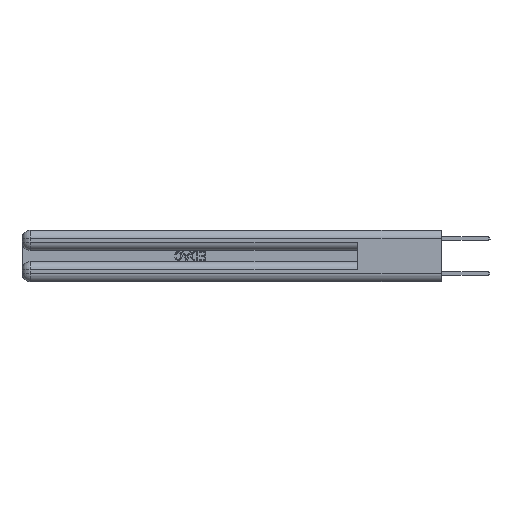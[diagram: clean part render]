
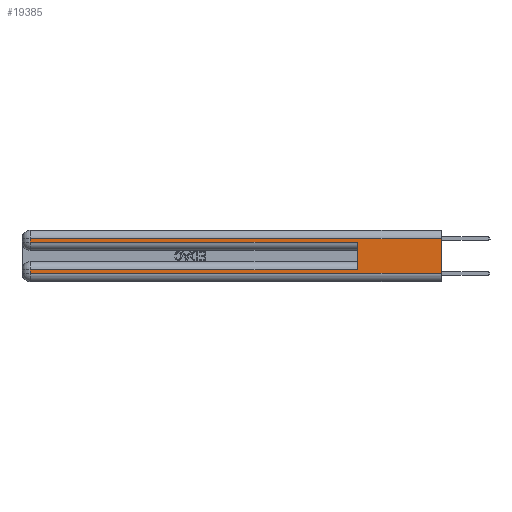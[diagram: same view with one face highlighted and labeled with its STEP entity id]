
A CAD part, left-side view. The second image highlights one B-rep face of the part: STEP entity #19385.
In plain terms, the highlighted planar face has unit normal (-1, 0, 0).
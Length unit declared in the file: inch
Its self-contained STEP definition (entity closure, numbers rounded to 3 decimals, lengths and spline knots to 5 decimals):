
#623 = CARTESIAN_POINT ( 'NONE',  ( 0., 0., 0.31 ) ) ;
#928 = ORIENTED_EDGE ( 'NONE', *, *, #11760, .T. ) ;
#1176 = LINE ( 'NONE', #1512, #12328 ) ;
#1384 = VERTEX_POINT ( 'NONE', #2148 ) ;
#1512 = CARTESIAN_POINT ( 'NONE',  ( 0., 2.94, 0.37 ) ) ;
#1855 = EDGE_CURVE ( 'NONE', #19437, #6624, #1176, .T. ) ;
#2148 = CARTESIAN_POINT ( 'NONE',  ( 0., 2.94, 0.085 ) ) ;
#2198 = DIRECTION ( 'NONE',  ( 0., 0., -1. ) ) ;
#2955 = DIRECTION ( 'NONE',  ( 0., 0., 1. ) ) ;
#3043 = ORIENTED_EDGE ( 'NONE', *, *, #7144, .T. ) ;
#3128 = FACE_OUTER_BOUND ( 'NONE', #19360, .T. ) ;
#3253 = ORIENTED_EDGE ( 'NONE', *, *, #17831, .F. ) ;
#3725 = DIRECTION ( 'NONE',  ( 0., 0., -1. ) ) ;
#3850 = VECTOR ( 'NONE', #22879, 39.37008 ) ;
#3863 = VERTEX_POINT ( 'NONE', #15389 ) ;
#3916 = LINE ( 'NONE', #19191, #9320 ) ;
#4671 = EDGE_CURVE ( 'NONE', #19615, #22689, #10793, .T. ) ;
#4676 = VECTOR ( 'NONE', #3725, 39.37008 ) ;
#4819 = ORIENTED_EDGE ( 'NONE', *, *, #1855, .T. ) ;
#6213 = CARTESIAN_POINT ( 'NONE',  ( 0., 0., 0.06 ) ) ;
#6471 = EDGE_CURVE ( 'NONE', #19615, #19437, #17158, .T. ) ;
#6624 = VERTEX_POINT ( 'NONE', #20461 ) ;
#7003 = CARTESIAN_POINT ( 'NONE',  ( 0., 2.94, 0.37 ) ) ;
#7045 = VECTOR ( 'NONE', #2198, 39.37008 ) ;
#7063 = EDGE_CURVE ( 'NONE', #12581, #22689, #22106, .T. ) ;
#7144 = EDGE_CURVE ( 'NONE', #1384, #12581, #22788, .T. ) ;
#8140 = VECTOR ( 'NONE', #27107, 39.37008 ) ;
#9320 = VECTOR ( 'NONE', #2955, 39.37008 ) ;
#9413 = VECTOR ( 'NONE', #19234, 39.37008 ) ;
#9540 = CARTESIAN_POINT ( 'NONE',  ( 0., 0., 0.085 ) ) ;
#10793 = LINE ( 'NONE', #12842, #4676 ) ;
#10964 = DIRECTION ( 'NONE',  ( 0., 0., -1. ) ) ;
#11760 = EDGE_CURVE ( 'NONE', #6624, #3863, #24926, .T. ) ;
#12117 = ORIENTED_EDGE ( 'NONE', *, *, #22693, .T. ) ;
#12328 = VECTOR ( 'NONE', #10964, 39.37008 ) ;
#12581 = VERTEX_POINT ( 'NONE', #21382 ) ;
#12842 = CARTESIAN_POINT ( 'NONE',  ( 0., 0., 0.37 ) ) ;
#13700 = ORIENTED_EDGE ( 'NONE', *, *, #7063, .T. ) ;
#15389 = CARTESIAN_POINT ( 'NONE',  ( 0., 0.6, 0.285 ) ) ;
#15562 = LINE ( 'NONE', #9540, #9413 ) ;
#15991 = DIRECTION ( 'NONE',  ( 1., 0., 0. ) ) ;
#16040 = CARTESIAN_POINT ( 'NONE',  ( 0., 0., 0.285 ) ) ;
#16197 = CARTESIAN_POINT ( 'NONE',  ( 0., 0., 0.37 ) ) ;
#17158 = LINE ( 'NONE', #29206, #8140 ) ;
#17831 = EDGE_CURVE ( 'NONE', #28899, #3863, #3916, .T. ) ;
#18501 = DIRECTION ( 'NONE',  ( 0., 0., -1. ) ) ;
#19032 = ORIENTED_EDGE ( 'NONE', *, *, #4671, .F. ) ;
#19191 = CARTESIAN_POINT ( 'NONE',  ( 0., 0.6, 0.145 ) ) ;
#19234 = DIRECTION ( 'NONE',  ( 0., 1., 0. ) ) ;
#19360 = EDGE_LOOP ( 'NONE', ( #19032, #20422, #4819, #928, #3253, #12117, #3043, #13700 ) ) ;
#19385 = ADVANCED_FACE ( 'NONE', ( #3128 ), #20872, .F. ) ;
#19437 = VERTEX_POINT ( 'NONE', #20756 ) ;
#19615 = VERTEX_POINT ( 'NONE', #623 ) ;
#19930 = AXIS2_PLACEMENT_3D ( 'NONE', #16197, #15991, #18501 ) ;
#19934 = DIRECTION ( 'NONE',  ( 0., -1., 0. ) ) ;
#20422 = ORIENTED_EDGE ( 'NONE', *, *, #6471, .T. ) ;
#20461 = CARTESIAN_POINT ( 'NONE',  ( 0., 2.94, 0.285 ) ) ;
#20756 = CARTESIAN_POINT ( 'NONE',  ( 0., 2.94, 0.31 ) ) ;
#20872 = PLANE ( 'NONE',  #19930 ) ;
#21382 = CARTESIAN_POINT ( 'NONE',  ( 0., 2.94, 0.06 ) ) ;
#22106 = LINE ( 'NONE', #6213, #24528 ) ;
#22689 = VERTEX_POINT ( 'NONE', #25161 ) ;
#22693 = EDGE_CURVE ( 'NONE', #28899, #1384, #15562, .T. ) ;
#22788 = LINE ( 'NONE', #7003, #7045 ) ;
#22796 = CARTESIAN_POINT ( 'NONE',  ( 0., 0.6, 0.085 ) ) ;
#22879 = DIRECTION ( 'NONE',  ( 0., -1., 0. ) ) ;
#24528 = VECTOR ( 'NONE', #19934, 39.37008 ) ;
#24926 = LINE ( 'NONE', #16040, #3850 ) ;
#25161 = CARTESIAN_POINT ( 'NONE',  ( 0., 0., 0.06 ) ) ;
#27107 = DIRECTION ( 'NONE',  ( 0., 1., 0. ) ) ;
#28899 = VERTEX_POINT ( 'NONE', #22796 ) ;
#29206 = CARTESIAN_POINT ( 'NONE',  ( 0., 0., 0.31 ) ) ;
